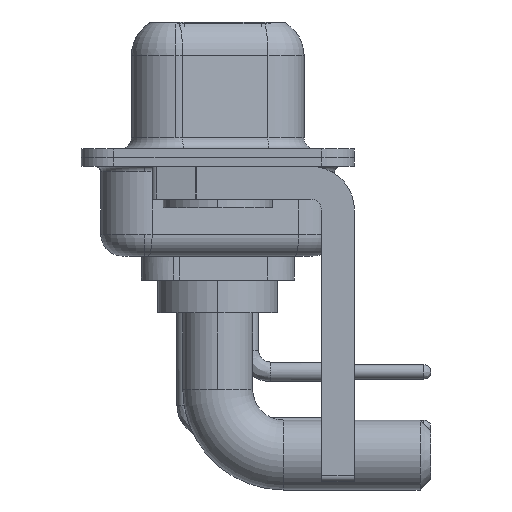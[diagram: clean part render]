
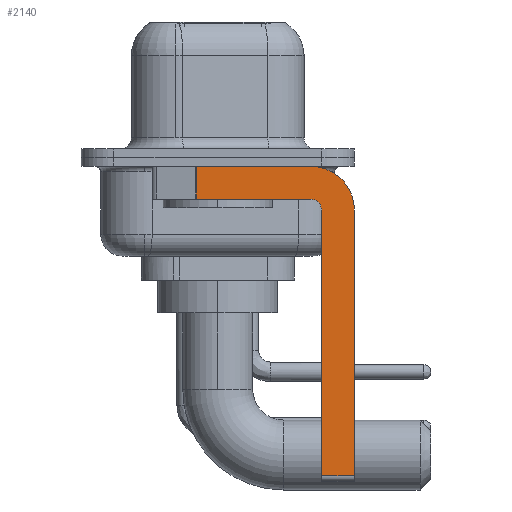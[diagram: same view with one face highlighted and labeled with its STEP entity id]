
A CAD part, left-side view. The second image highlights one B-rep face of the part: STEP entity #2140.
In plain terms, the highlighted planar face has unit normal (-1, 0, 0).
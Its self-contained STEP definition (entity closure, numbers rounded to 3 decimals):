
#179 = CARTESIAN_POINT ( 'NONE',  ( -2.9, -4.75, -2.4 ) ) ;
#1030 = VECTOR ( 'NONE', #10685, 1000. ) ;
#1199 = DIRECTION ( 'NONE',  ( 0., -1., 0. ) ) ;
#1439 = CARTESIAN_POINT ( 'NONE',  ( -2.9, -4.25, -14.55 ) ) ;
#1857 = VECTOR ( 'NONE', #5293, 1000. ) ;
#1904 = EDGE_CURVE ( 'NONE', #2570, #17913, #16536, .T. ) ;
#2140 = ADVANCED_FACE ( 'NONE', ( #2741 ), #4199, .F. ) ;
#2196 = VERTEX_POINT ( 'NONE', #16717 ) ;
#2379 = CARTESIAN_POINT ( 'NONE',  ( -2.9, -4.25, -2.4 ) ) ;
#2570 = VERTEX_POINT ( 'NONE', #179 ) ;
#2741 = FACE_OUTER_BOUND ( 'NONE', #8815, .T. ) ;
#2833 = AXIS2_PLACEMENT_3D ( 'NONE', #9777, #15334, #15150 ) ;
#3085 = CARTESIAN_POINT ( 'NONE',  ( -2.9, -4.75, -14.8 ) ) ;
#3523 = VERTEX_POINT ( 'NONE', #10621 ) ;
#3865 = ORIENTED_EDGE ( 'NONE', *, *, #1904, .F. ) ;
#4199 = PLANE ( 'NONE',  #2833 ) ;
#4455 = CARTESIAN_POINT ( 'NONE',  ( -2.9, -4.25, -2.4 ) ) ;
#4538 = EDGE_CURVE ( 'NONE', #17278, #7342, #15295, .T. ) ;
#4685 = DIRECTION ( 'NONE',  ( 0., -1., 0. ) ) ;
#5293 = DIRECTION ( 'NONE',  ( 0., 0., -1. ) ) ;
#5484 = LINE ( 'NONE', #11053, #1030 ) ;
#5552 = ORIENTED_EDGE ( 'NONE', *, *, #9931, .F. ) ;
#6396 = VECTOR ( 'NONE', #4685, 1000. ) ;
#6674 = CARTESIAN_POINT ( 'NONE',  ( -2.9, -4.25, -0.4 ) ) ;
#6687 = CARTESIAN_POINT ( 'NONE',  ( -2.9, -6.25, -2.4 ) ) ;
#6741 = VECTOR ( 'NONE', #10210, 1000. ) ;
#6852 = VECTOR ( 'NONE', #1199, 1000. ) ;
#7013 = VERTEX_POINT ( 'NONE', #6674 ) ;
#7342 = VERTEX_POINT ( 'NONE', #7388 ) ;
#7388 = CARTESIAN_POINT ( 'NONE',  ( -2.9, -6.25, -14.55 ) ) ;
#7769 = ORIENTED_EDGE ( 'NONE', *, *, #15866, .F. ) ;
#7797 = ORIENTED_EDGE ( 'NONE', *, *, #4538, .T. ) ;
#7845 = EDGE_CURVE ( 'NONE', #17278, #2570, #12945, .T. ) ;
#7934 = DIRECTION ( 'NONE',  ( 0., 0., 1. ) ) ;
#8126 = LINE ( 'NONE', #17721, #1857 ) ;
#8802 = CARTESIAN_POINT ( 'NONE',  ( -2.9, -6.25, -2.4 ) ) ;
#8815 = EDGE_LOOP ( 'NONE', ( #11113, #14155, #15000, #3865, #9555, #7797, #7769, #5552 ) ) ;
#9555 = ORIENTED_EDGE ( 'NONE', *, *, #7845, .F. ) ;
#9777 = CARTESIAN_POINT ( 'NONE',  ( -2.9, -4.25, -2.4 ) ) ;
#9931 = EDGE_CURVE ( 'NONE', #7013, #11617, #13177, .T. ) ;
#10113 = AXIS2_PLACEMENT_3D ( 'NONE', #2379, #13783, #7934 ) ;
#10210 = DIRECTION ( 'NONE',  ( 0., 0., 1. ) ) ;
#10621 = CARTESIAN_POINT ( 'NONE',  ( -2.9, 0.978, -1.9 ) ) ;
#10685 = DIRECTION ( 'NONE',  ( 0., 1., 0. ) ) ;
#10912 = VECTOR ( 'NONE', #12257, 1000. ) ;
#11053 = CARTESIAN_POINT ( 'NONE',  ( -2.9, -4.25, -1.9 ) ) ;
#11113 = ORIENTED_EDGE ( 'NONE', *, *, #16984, .F. ) ;
#11221 = DIRECTION ( 'NONE',  ( 0., 0., -1. ) ) ;
#11617 = VERTEX_POINT ( 'NONE', #8802 ) ;
#12018 = AXIS2_PLACEMENT_3D ( 'NONE', #4455, #12585, #11221 ) ;
#12257 = DIRECTION ( 'NONE',  ( 0., 0., -1. ) ) ;
#12353 = LINE ( 'NONE', #6687, #10912 ) ;
#12585 = DIRECTION ( 'NONE',  ( 1., 0., 0. ) ) ;
#12945 = LINE ( 'NONE', #3085, #6741 ) ;
#13177 = CIRCLE ( 'NONE', #12018, 2. ) ;
#13783 = DIRECTION ( 'NONE',  ( -1., 0., 0. ) ) ;
#14155 = ORIENTED_EDGE ( 'NONE', *, *, #14851, .T. ) ;
#14851 = EDGE_CURVE ( 'NONE', #2196, #3523, #8126, .T. ) ;
#15000 = ORIENTED_EDGE ( 'NONE', *, *, #16298, .F. ) ;
#15150 = DIRECTION ( 'NONE',  ( 0., 0., -1. ) ) ;
#15295 = LINE ( 'NONE', #1439, #6396 ) ;
#15329 = CARTESIAN_POINT ( 'NONE',  ( -2.9, -4.75, -14.55 ) ) ;
#15334 = DIRECTION ( 'NONE',  ( 1., 0., 0. ) ) ;
#15866 = EDGE_CURVE ( 'NONE', #11617, #7342, #12353, .T. ) ;
#16298 = EDGE_CURVE ( 'NONE', #17913, #3523, #5484, .T. ) ;
#16536 = CIRCLE ( 'NONE', #10113, 0.5 ) ;
#16717 = CARTESIAN_POINT ( 'NONE',  ( -2.9, 0.978, -0.4 ) ) ;
#16984 = EDGE_CURVE ( 'NONE', #2196, #7013, #17801, .T. ) ;
#17224 = CARTESIAN_POINT ( 'NONE',  ( -2.9, -4.25, -1.9 ) ) ;
#17278 = VERTEX_POINT ( 'NONE', #15329 ) ;
#17624 = CARTESIAN_POINT ( 'NONE',  ( -2.9, 3., -0.4 ) ) ;
#17721 = CARTESIAN_POINT ( 'NONE',  ( -2.9, 0.978, -1.9 ) ) ;
#17801 = LINE ( 'NONE', #17624, #6852 ) ;
#17913 = VERTEX_POINT ( 'NONE', #17224 ) ;
